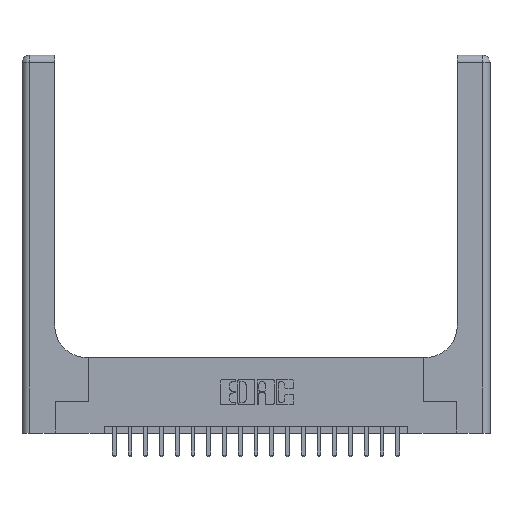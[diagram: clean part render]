
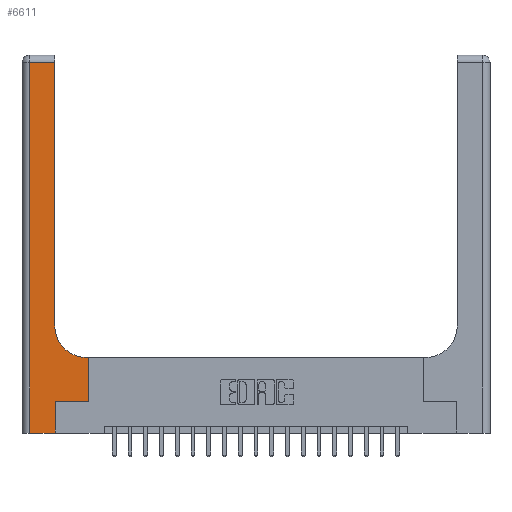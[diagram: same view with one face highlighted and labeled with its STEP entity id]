
A CAD part, top view. The second image highlights one B-rep face of the part: STEP entity #6611.
In plain terms, the highlighted planar face has unit normal (0, 0, 1).
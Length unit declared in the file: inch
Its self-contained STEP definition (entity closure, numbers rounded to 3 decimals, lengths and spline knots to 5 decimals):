
#871 = CARTESIAN_POINT ( 'NONE',  ( 0., 2.94, 0.37 ) ) ;
#919 = CARTESIAN_POINT ( 'NONE',  ( 0.26, 0.6, 0.37 ) ) ;
#937 = CARTESIAN_POINT ( 'NONE',  ( 0.265, 0.25, 0.37 ) ) ;
#1080 = DIRECTION ( 'NONE',  ( 1., 0., 0. ) ) ;
#1157 = DIRECTION ( 'NONE',  ( 1., 0., 0. ) ) ;
#1293 = LINE ( 'NONE', #919, #13115 ) ;
#1509 = EDGE_CURVE ( 'NONE', #5164, #4203, #16457, .T. ) ;
#1536 = VERTEX_POINT ( 'NONE', #4871 ) ;
#1594 = DIRECTION ( 'NONE',  ( 0., 1., 0. ) ) ;
#1735 = EDGE_CURVE ( 'NONE', #16752, #9708, #7926, .T. ) ;
#2330 = CARTESIAN_POINT ( 'NONE',  ( 0.51, 0.6, 0.37 ) ) ;
#2549 = CARTESIAN_POINT ( 'NONE',  ( 0.06, 0., 0.37 ) ) ;
#2618 = CIRCLE ( 'NONE', #11367, 0.25 ) ;
#4001 = LINE ( 'NONE', #937, #15823 ) ;
#4169 = ORIENTED_EDGE ( 'NONE', *, *, #18559, .T. ) ;
#4187 = AXIS2_PLACEMENT_3D ( 'NONE', #9342, #18948, #12339 ) ;
#4203 = VERTEX_POINT ( 'NONE', #20354 ) ;
#4871 = CARTESIAN_POINT ( 'NONE',  ( 0.265, 0., 0.37 ) ) ;
#5164 = VERTEX_POINT ( 'NONE', #13610 ) ;
#5391 = ORIENTED_EDGE ( 'NONE', *, *, #15807, .T. ) ;
#5746 = CARTESIAN_POINT ( 'NONE',  ( 0., 0., 0.37 ) ) ;
#6160 = EDGE_CURVE ( 'NONE', #1536, #14525, #19363, .T. ) ;
#6496 = CARTESIAN_POINT ( 'NONE',  ( 0.51, 0.85, 0.37 ) ) ;
#6554 = VERTEX_POINT ( 'NONE', #18524 ) ;
#6611 = ADVANCED_FACE ( 'NONE', ( #15313 ), #12484, .F. ) ;
#6719 = EDGE_LOOP ( 'NONE', ( #11587, #11052, #10915, #5391, #11428, #19701, #10300, #4169, #9685 ) ) ;
#7642 = EDGE_CURVE ( 'NONE', #9708, #9298, #12272, .T. ) ;
#7841 = CARTESIAN_POINT ( 'NONE',  ( 0.06, 2.94, 0.37 ) ) ;
#7926 = LINE ( 'NONE', #871, #20691 ) ;
#8144 = CARTESIAN_POINT ( 'NONE',  ( 0.528, 0.25, 0.37 ) ) ;
#8725 = CARTESIAN_POINT ( 'NONE',  ( 0.26, 3., 0.37 ) ) ;
#9298 = VERTEX_POINT ( 'NONE', #2549 ) ;
#9342 = CARTESIAN_POINT ( 'NONE',  ( 0., 3., 0.37 ) ) ;
#9584 = DIRECTION ( 'NONE',  ( 0., 0., -1. ) ) ;
#9685 = ORIENTED_EDGE ( 'NONE', *, *, #9845, .T. ) ;
#9708 = VERTEX_POINT ( 'NONE', #7841 ) ;
#9843 = VECTOR ( 'NONE', #1080, 39.37008 ) ;
#9845 = EDGE_CURVE ( 'NONE', #19017, #6554, #2618, .T. ) ;
#10300 = ORIENTED_EDGE ( 'NONE', *, *, #1509, .T. ) ;
#10674 = VECTOR ( 'NONE', #18033, 39.37008 ) ;
#10915 = ORIENTED_EDGE ( 'NONE', *, *, #7642, .T. ) ;
#11052 = ORIENTED_EDGE ( 'NONE', *, *, #1735, .T. ) ;
#11117 = CARTESIAN_POINT ( 'NONE',  ( 0.265, 0., 0.37 ) ) ;
#11367 = AXIS2_PLACEMENT_3D ( 'NONE', #6496, #9584, #12855 ) ;
#11428 = ORIENTED_EDGE ( 'NONE', *, *, #6160, .T. ) ;
#11587 = ORIENTED_EDGE ( 'NONE', *, *, #17753, .T. ) ;
#11702 = DIRECTION ( 'NONE',  ( 0., 1., 0. ) ) ;
#12272 = LINE ( 'NONE', #12398, #19538 ) ;
#12339 = DIRECTION ( 'NONE',  ( -1., 0., 0. ) ) ;
#12398 = CARTESIAN_POINT ( 'NONE',  ( 0.06, 3., 0.37 ) ) ;
#12484 = PLANE ( 'NONE',  #4187 ) ;
#12855 = DIRECTION ( 'NONE',  ( 1., 0., 0. ) ) ;
#13115 = VECTOR ( 'NONE', #13905, 39.37008 ) ;
#13274 = LINE ( 'NONE', #8725, #14538 ) ;
#13610 = CARTESIAN_POINT ( 'NONE',  ( 0.528, 0.25, 0.37 ) ) ;
#13905 = DIRECTION ( 'NONE',  ( -1., 0., 0. ) ) ;
#14087 = LINE ( 'NONE', #5746, #9843 ) ;
#14135 = DIRECTION ( 'NONE',  ( 0., -1., 0. ) ) ;
#14525 = VERTEX_POINT ( 'NONE', #16658 ) ;
#14538 = VECTOR ( 'NONE', #11702, 39.37008 ) ;
#15313 = FACE_OUTER_BOUND ( 'NONE', #6719, .T. ) ;
#15807 = EDGE_CURVE ( 'NONE', #9298, #1536, #14087, .T. ) ;
#15823 = VECTOR ( 'NONE', #1157, 39.37008 ) ;
#16100 = VECTOR ( 'NONE', #1594, 39.37008 ) ;
#16333 = EDGE_CURVE ( 'NONE', #14525, #5164, #4001, .T. ) ;
#16457 = LINE ( 'NONE', #8144, #10674 ) ;
#16463 = DIRECTION ( 'NONE',  ( -1., 0., 0. ) ) ;
#16658 = CARTESIAN_POINT ( 'NONE',  ( 0.265, 0.25, 0.37 ) ) ;
#16752 = VERTEX_POINT ( 'NONE', #18557 ) ;
#17753 = EDGE_CURVE ( 'NONE', #6554, #16752, #13274, .T. ) ;
#18033 = DIRECTION ( 'NONE',  ( 0., 1., 0. ) ) ;
#18524 = CARTESIAN_POINT ( 'NONE',  ( 0.26, 0.85, 0.37 ) ) ;
#18557 = CARTESIAN_POINT ( 'NONE',  ( 0.26, 2.94, 0.37 ) ) ;
#18559 = EDGE_CURVE ( 'NONE', #4203, #19017, #1293, .T. ) ;
#18948 = DIRECTION ( 'NONE',  ( 0., 0., -1. ) ) ;
#19017 = VERTEX_POINT ( 'NONE', #2330 ) ;
#19363 = LINE ( 'NONE', #11117, #16100 ) ;
#19538 = VECTOR ( 'NONE', #14135, 39.37008 ) ;
#19701 = ORIENTED_EDGE ( 'NONE', *, *, #16333, .T. ) ;
#20354 = CARTESIAN_POINT ( 'NONE',  ( 0.528, 0.6, 0.37 ) ) ;
#20691 = VECTOR ( 'NONE', #16463, 39.37008 ) ;
